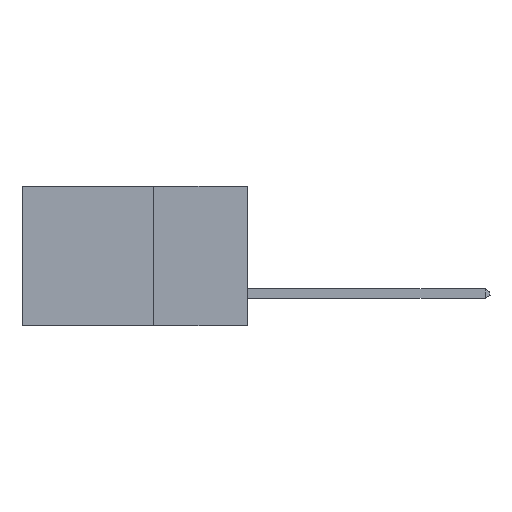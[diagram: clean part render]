
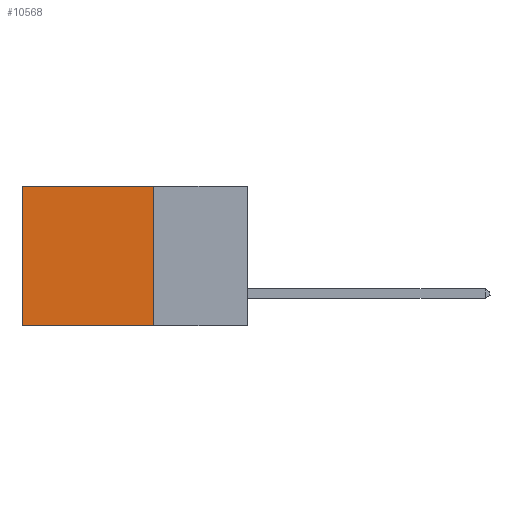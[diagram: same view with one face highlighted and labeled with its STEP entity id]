
A CAD part, left-side view. The second image highlights one B-rep face of the part: STEP entity #10568.
In plain terms, the highlighted planar face has unit normal (-1, 0, 0).
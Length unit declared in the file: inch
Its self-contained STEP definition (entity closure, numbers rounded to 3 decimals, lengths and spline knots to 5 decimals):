
#69 = EDGE_LOOP ( 'NONE', ( #2997, #7345, #1711, #9844 ) ) ;
#420 = CARTESIAN_POINT ( 'NONE',  ( 0.298, 0.6, 0. ) ) ;
#1087 = FACE_OUTER_BOUND ( 'NONE', #69, .T. ) ;
#1588 = DIRECTION ( 'NONE',  ( 0., 0., -1. ) ) ;
#1615 = VECTOR ( 'NONE', #8472, 39.37008 ) ;
#1675 = VECTOR ( 'NONE', #2215, 39.37008 ) ;
#1711 = ORIENTED_EDGE ( 'NONE', *, *, #3799, .F. ) ;
#2157 = CARTESIAN_POINT ( 'NONE',  ( 0.298, 0.25, 0. ) ) ;
#2215 = DIRECTION ( 'NONE',  ( 0., 0., -1. ) ) ;
#2271 = LINE ( 'NONE', #4048, #6779 ) ;
#2278 = VERTEX_POINT ( 'NONE', #3472 ) ;
#2581 = LINE ( 'NONE', #6680, #1615 ) ;
#2997 = ORIENTED_EDGE ( 'NONE', *, *, #10092, .T. ) ;
#3472 = CARTESIAN_POINT ( 'NONE',  ( 0.298, 0.6, -0.37 ) ) ;
#3799 = EDGE_CURVE ( 'NONE', #8943, #9232, #2581, .T. ) ;
#4048 = CARTESIAN_POINT ( 'NONE',  ( 0.298, 0.25, -0.37 ) ) ;
#4421 = VERTEX_POINT ( 'NONE', #4509 ) ;
#4509 = CARTESIAN_POINT ( 'NONE',  ( 0.298, 0.6, 0. ) ) ;
#5181 = CARTESIAN_POINT ( 'NONE',  ( 0.298, 0.25, 0. ) ) ;
#5252 = DIRECTION ( 'NONE',  ( 1., 0., 0. ) ) ;
#5333 = CARTESIAN_POINT ( 'NONE',  ( 0.298, 0.25, 0. ) ) ;
#5758 = LINE ( 'NONE', #5333, #8555 ) ;
#6034 = PLANE ( 'NONE',  #9169 ) ;
#6680 = CARTESIAN_POINT ( 'NONE',  ( 0.298, 0.25, 0. ) ) ;
#6779 = VECTOR ( 'NONE', #7655, 39.37008 ) ;
#7345 = ORIENTED_EDGE ( 'NONE', *, *, #7876, .F. ) ;
#7655 = DIRECTION ( 'NONE',  ( 0., 1., 0. ) ) ;
#7876 = EDGE_CURVE ( 'NONE', #9232, #2278, #2271, .T. ) ;
#8472 = DIRECTION ( 'NONE',  ( 0., 0., -1. ) ) ;
#8555 = VECTOR ( 'NONE', #11567, 39.37008 ) ;
#8943 = VERTEX_POINT ( 'NONE', #2157 ) ;
#9169 = AXIS2_PLACEMENT_3D ( 'NONE', #5181, #5252, #1588 ) ;
#9232 = VERTEX_POINT ( 'NONE', #11054 ) ;
#9686 = EDGE_CURVE ( 'NONE', #8943, #4421, #5758, .T. ) ;
#9844 = ORIENTED_EDGE ( 'NONE', *, *, #9686, .T. ) ;
#10092 = EDGE_CURVE ( 'NONE', #4421, #2278, #11207, .T. ) ;
#10568 = ADVANCED_FACE ( 'NONE', ( #1087 ), #6034, .F. ) ;
#11054 = CARTESIAN_POINT ( 'NONE',  ( 0.298, 0.25, -0.37 ) ) ;
#11207 = LINE ( 'NONE', #420, #1675 ) ;
#11567 = DIRECTION ( 'NONE',  ( 0., 1., 0. ) ) ;
